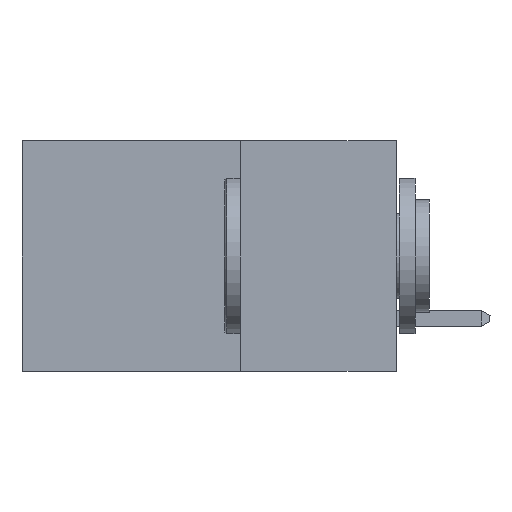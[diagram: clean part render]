
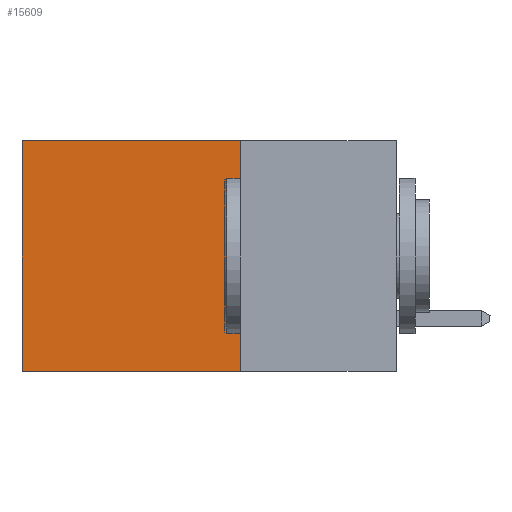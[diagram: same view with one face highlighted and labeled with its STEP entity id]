
A CAD part, left-side view. The second image highlights one B-rep face of the part: STEP entity #15609.
In plain terms, the highlighted planar face has unit normal (-1, 0, 0).
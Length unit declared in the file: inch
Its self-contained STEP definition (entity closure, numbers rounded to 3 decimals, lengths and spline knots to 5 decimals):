
#484 = VECTOR ( 'NONE', #776, 39.37008 ) ;
#776 = DIRECTION ( 'NONE',  ( 0., 0., -1. ) ) ;
#3555 = EDGE_CURVE ( 'NONE', #23051, #19764, #10692, .T. ) ;
#3965 = VECTOR ( 'NONE', #13360, 39.37008 ) ;
#3985 = ORIENTED_EDGE ( 'NONE', *, *, #19275, .F. ) ;
#4581 = AXIS2_PLACEMENT_3D ( 'NONE', #20340, #14319, #8352 ) ;
#5563 = VERTEX_POINT ( 'NONE', #25503 ) ;
#5653 = ORIENTED_EDGE ( 'NONE', *, *, #5660, .T. ) ;
#5660 = EDGE_CURVE ( 'NONE', #5563, #8839, #17881, .T. ) ;
#5912 = FACE_OUTER_BOUND ( 'NONE', #22753, .T. ) ;
#6180 = EDGE_CURVE ( 'NONE', #23051, #5563, #9284, .T. ) ;
#6631 = ORIENTED_EDGE ( 'NONE', *, *, #3555, .F. ) ;
#8352 = DIRECTION ( 'NONE',  ( 0., 0., -1. ) ) ;
#8839 = VERTEX_POINT ( 'NONE', #21708 ) ;
#9284 = LINE ( 'NONE', #11200, #3965 ) ;
#10692 = LINE ( 'NONE', #19124, #21515 ) ;
#11031 = LINE ( 'NONE', #19618, #22512 ) ;
#11200 = CARTESIAN_POINT ( 'NONE',  ( 0.2615, 0.25, 0. ) ) ;
#13360 = DIRECTION ( 'NONE',  ( 0., 1., 0. ) ) ;
#14319 = DIRECTION ( 'NONE',  ( 1., 0., 0. ) ) ;
#14581 = PLANE ( 'NONE',  #4581 ) ;
#15609 = ADVANCED_FACE ( 'NONE', ( #5912 ), #14581, .F. ) ;
#17881 = LINE ( 'NONE', #26169, #484 ) ;
#18989 = DIRECTION ( 'NONE',  ( 0., 0., -1. ) ) ;
#19124 = CARTESIAN_POINT ( 'NONE',  ( 0.2615, 0.25, -0.37 ) ) ;
#19275 = EDGE_CURVE ( 'NONE', #19764, #8839, #11031, .T. ) ;
#19570 = CARTESIAN_POINT ( 'NONE',  ( 0.2615, 0.25, 0. ) ) ;
#19618 = CARTESIAN_POINT ( 'NONE',  ( 0.2615, 0.25, -0.37 ) ) ;
#19764 = VERTEX_POINT ( 'NONE', #23891 ) ;
#20340 = CARTESIAN_POINT ( 'NONE',  ( 0.2615, 0.25, -0.37 ) ) ;
#21515 = VECTOR ( 'NONE', #18989, 39.37008 ) ;
#21646 = DIRECTION ( 'NONE',  ( 0., 1., 0. ) ) ;
#21708 = CARTESIAN_POINT ( 'NONE',  ( 0.2615, 0.6, -0.37 ) ) ;
#22512 = VECTOR ( 'NONE', #21646, 39.37008 ) ;
#22753 = EDGE_LOOP ( 'NONE', ( #5653, #3985, #6631, #26790 ) ) ;
#23051 = VERTEX_POINT ( 'NONE', #19570 ) ;
#23891 = CARTESIAN_POINT ( 'NONE',  ( 0.2615, 0.25, -0.37 ) ) ;
#25503 = CARTESIAN_POINT ( 'NONE',  ( 0.2615, 0.6, 0. ) ) ;
#26169 = CARTESIAN_POINT ( 'NONE',  ( 0.2615, 0.6, -0.37 ) ) ;
#26790 = ORIENTED_EDGE ( 'NONE', *, *, #6180, .T. ) ;
